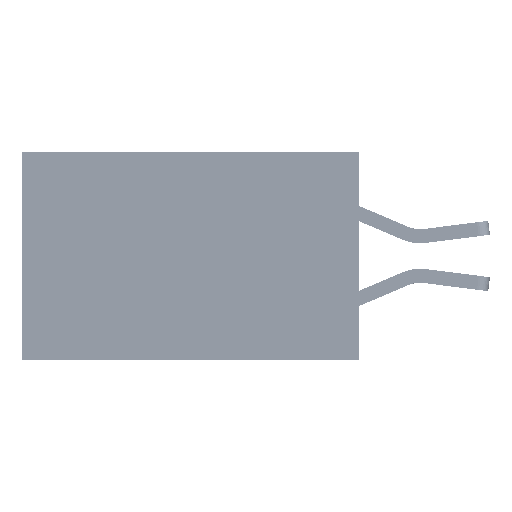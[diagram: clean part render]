
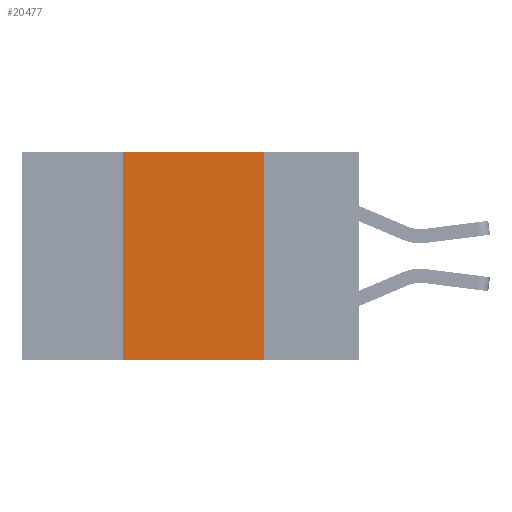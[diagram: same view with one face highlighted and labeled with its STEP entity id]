
A CAD part, left-side view. The second image highlights one B-rep face of the part: STEP entity #20477.
In plain terms, the highlighted planar face has unit normal (-1, 0, 0).
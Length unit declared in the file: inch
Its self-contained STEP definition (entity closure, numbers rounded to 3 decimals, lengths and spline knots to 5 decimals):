
#67 = PLANE ( 'NONE',  #31577 ) ;
#1623 = EDGE_CURVE ( 'NONE', #4789, #9710, #1653, .T. ) ;
#1653 = LINE ( 'NONE', #25272, #9743 ) ;
#2805 = CARTESIAN_POINT ( 'NONE',  ( 0., 0.17, -0.37 ) ) ;
#2957 = LINE ( 'NONE', #45586, #20762 ) ;
#3282 = VERTEX_POINT ( 'NONE', #35132 ) ;
#3566 = ORIENTED_EDGE ( 'NONE', *, *, #23556, .F. ) ;
#3812 = ORIENTED_EDGE ( 'NONE', *, *, #44668, .F. ) ;
#4789 = VERTEX_POINT ( 'NONE', #46575 ) ;
#6623 = CARTESIAN_POINT ( 'NONE',  ( 0., 0.6, 0. ) ) ;
#9710 = VERTEX_POINT ( 'NONE', #2805 ) ;
#9743 = VECTOR ( 'NONE', #36415, 39.37008 ) ;
#10818 = DIRECTION ( 'NONE',  ( 0., 0., 1. ) ) ;
#13243 = VECTOR ( 'NONE', #25893, 39.37008 ) ;
#13952 = LINE ( 'NONE', #6623, #21719 ) ;
#14774 = DIRECTION ( 'NONE',  ( 1., 0., 0. ) ) ;
#18846 = DIRECTION ( 'NONE',  ( 0., 0., -1. ) ) ;
#20477 = ADVANCED_FACE ( 'NONE', ( #38631 ), #67, .F. ) ;
#20502 = VERTEX_POINT ( 'NONE', #41678 ) ;
#20762 = VECTOR ( 'NONE', #10818, 39.37008 ) ;
#21719 = VECTOR ( 'NONE', #29465, 39.37008 ) ;
#23556 = EDGE_CURVE ( 'NONE', #20502, #3282, #13952, .T. ) ;
#25272 = CARTESIAN_POINT ( 'NONE',  ( 0., 0.6, -0.37 ) ) ;
#25893 = DIRECTION ( 'NONE',  ( 0., 0., -1. ) ) ;
#29465 = DIRECTION ( 'NONE',  ( 0., -1., 0. ) ) ;
#31042 = CARTESIAN_POINT ( 'NONE',  ( 0., 0.6, 0. ) ) ;
#31577 = AXIS2_PLACEMENT_3D ( 'NONE', #31042, #14774, #18846 ) ;
#35132 = CARTESIAN_POINT ( 'NONE',  ( 0., 0.17, 0. ) ) ;
#36362 = ORIENTED_EDGE ( 'NONE', *, *, #1623, .T. ) ;
#36415 = DIRECTION ( 'NONE',  ( 0., -1., 0. ) ) ;
#38631 = FACE_OUTER_BOUND ( 'NONE', #43648, .T. ) ;
#41074 = LINE ( 'NONE', #41579, #13243 ) ;
#41579 = CARTESIAN_POINT ( 'NONE',  ( 0., 0.17, 0. ) ) ;
#41678 = CARTESIAN_POINT ( 'NONE',  ( 0., 0.42, 0. ) ) ;
#43648 = EDGE_LOOP ( 'NONE', ( #3812, #3566, #45452, #36362 ) ) ;
#44668 = EDGE_CURVE ( 'NONE', #3282, #9710, #41074, .T. ) ;
#45452 = ORIENTED_EDGE ( 'NONE', *, *, #47921, .F. ) ;
#45586 = CARTESIAN_POINT ( 'NONE',  ( 0., 0.42, 0. ) ) ;
#46575 = CARTESIAN_POINT ( 'NONE',  ( 0., 0.42, -0.37 ) ) ;
#47921 = EDGE_CURVE ( 'NONE', #4789, #20502, #2957, .T. ) ;
